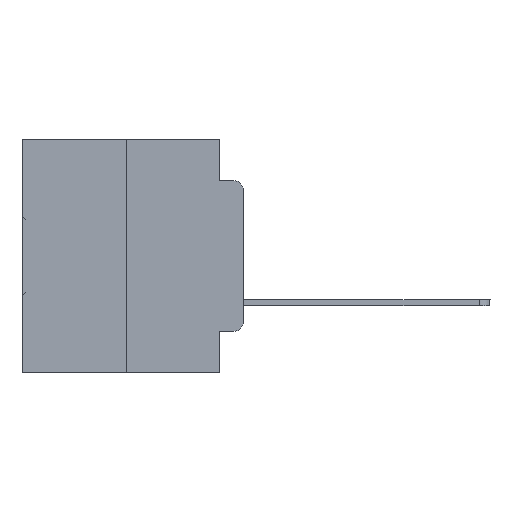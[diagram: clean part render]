
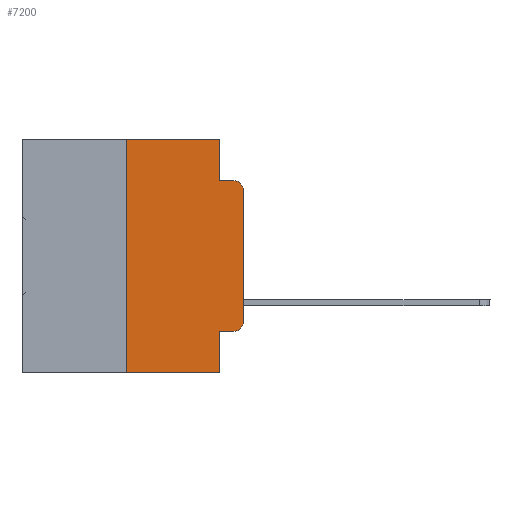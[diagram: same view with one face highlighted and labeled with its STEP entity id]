
A CAD part, left-side view. The second image highlights one B-rep face of the part: STEP entity #7200.
In plain terms, the highlighted planar face has unit normal (-1, 0, 0).
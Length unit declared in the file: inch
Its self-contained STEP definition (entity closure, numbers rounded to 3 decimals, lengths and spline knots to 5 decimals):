
#380 = DIRECTION ( 'NONE',  ( 0., 0., -1. ) ) ;
#623 = VECTOR ( 'NONE', #21628, 39.37008 ) ;
#686 = CARTESIAN_POINT ( 'NONE',  ( 0., 0.02, -0.3915 ) ) ;
#1018 = ORIENTED_EDGE ( 'NONE', *, *, #17901, .F. ) ;
#1447 = DIRECTION ( 'NONE',  ( 0., -1., 0. ) ) ;
#1550 = FACE_OUTER_BOUND ( 'NONE', #14288, .T. ) ;
#1803 = CARTESIAN_POINT ( 'NONE',  ( 0., 0.051, -0.4115 ) ) ;
#2067 = DIRECTION ( 'NONE',  ( 0., 0., -1. ) ) ;
#2581 = CARTESIAN_POINT ( 'NONE',  ( 0., 0.051, 0. ) ) ;
#2599 = CARTESIAN_POINT ( 'NONE',  ( 0., 0.051, 0. ) ) ;
#2606 = CARTESIAN_POINT ( 'NONE',  ( 0., 0.051, -0.0885 ) ) ;
#2809 = VERTEX_POINT ( 'NONE', #28054 ) ;
#3084 = DIRECTION ( 'NONE',  ( -1., 0., 0. ) ) ;
#3842 = CARTESIAN_POINT ( 'NONE',  ( 0., 0., -0.3915 ) ) ;
#4017 = EDGE_CURVE ( 'NONE', #8061, #31795, #25073, .T. ) ;
#4572 = DIRECTION ( 'NONE',  ( 1., 0., 0. ) ) ;
#4584 = EDGE_CURVE ( 'NONE', #8061, #24535, #31628, .T. ) ;
#4909 = CARTESIAN_POINT ( 'NONE',  ( 0., 0.473, 0. ) ) ;
#5187 = LINE ( 'NONE', #12226, #9756 ) ;
#5697 = ORIENTED_EDGE ( 'NONE', *, *, #12408, .T. ) ;
#5806 = CARTESIAN_POINT ( 'NONE',  ( 0., 0.473, -0.5 ) ) ;
#6037 = EDGE_CURVE ( 'NONE', #8994, #27516, #20230, .T. ) ;
#6331 = CARTESIAN_POINT ( 'NONE',  ( 0., 0.051, -0.4115 ) ) ;
#7171 = EDGE_CURVE ( 'NONE', #12189, #2809, #15209, .T. ) ;
#7200 = ADVANCED_FACE ( 'NONE', ( #1550 ), #25599, .F. ) ;
#7308 = CARTESIAN_POINT ( 'NONE',  ( 0., 0.051, 0. ) ) ;
#7859 = ORIENTED_EDGE ( 'NONE', *, *, #6037, .F. ) ;
#8061 = VERTEX_POINT ( 'NONE', #6331 ) ;
#8823 = ORIENTED_EDGE ( 'NONE', *, *, #29715, .F. ) ;
#8994 = VERTEX_POINT ( 'NONE', #2599 ) ;
#9609 = CIRCLE ( 'NONE', #23809, 0.02 ) ;
#9756 = VECTOR ( 'NONE', #14757, 39.37008 ) ;
#9885 = DIRECTION ( 'NONE',  ( 0., 0., 1. ) ) ;
#11040 = VECTOR ( 'NONE', #1447, 39.37008 ) ;
#11096 = CARTESIAN_POINT ( 'NONE',  ( 0., 0.051, -0.5 ) ) ;
#11649 = ORIENTED_EDGE ( 'NONE', *, *, #7171, .T. ) ;
#12012 = ORIENTED_EDGE ( 'NONE', *, *, #4584, .F. ) ;
#12189 = VERTEX_POINT ( 'NONE', #30279 ) ;
#12226 = CARTESIAN_POINT ( 'NONE',  ( 0., 0.25, 0. ) ) ;
#12408 = EDGE_CURVE ( 'NONE', #15533, #12189, #27137, .T. ) ;
#13996 = CARTESIAN_POINT ( 'NONE',  ( 0., 0.25, 0. ) ) ;
#14288 = EDGE_LOOP ( 'NONE', ( #5697, #11649, #30244, #7859, #8823, #1018, #22635, #12012, #19996, #14322 ) ) ;
#14322 = ORIENTED_EDGE ( 'NONE', *, *, #24398, .T. ) ;
#14585 = VERTEX_POINT ( 'NONE', #13996 ) ;
#14757 = DIRECTION ( 'NONE',  ( 0., 0., 1. ) ) ;
#15209 = CIRCLE ( 'NONE', #17328, 0.02 ) ;
#15533 = VERTEX_POINT ( 'NONE', #3842 ) ;
#16756 = EDGE_CURVE ( 'NONE', #33252, #24535, #29791, .T. ) ;
#17328 = AXIS2_PLACEMENT_3D ( 'NONE', #28610, #18133, #28371 ) ;
#17901 = EDGE_CURVE ( 'NONE', #33252, #14585, #5187, .T. ) ;
#18133 = DIRECTION ( 'NONE',  ( -1., 0., 0. ) ) ;
#18257 = EDGE_CURVE ( 'NONE', #27516, #2809, #27036, .T. ) ;
#18319 = CARTESIAN_POINT ( 'NONE',  ( 0., 0.473, 0. ) ) ;
#19069 = AXIS2_PLACEMENT_3D ( 'NONE', #4909, #4572, #2067 ) ;
#19996 = ORIENTED_EDGE ( 'NONE', *, *, #4017, .T. ) ;
#20225 = VECTOR ( 'NONE', #31537, 39.37008 ) ;
#20230 = LINE ( 'NONE', #2581, #26422 ) ;
#21628 = DIRECTION ( 'NONE',  ( 0., -1., 0. ) ) ;
#21705 = VECTOR ( 'NONE', #33289, 39.37008 ) ;
#22635 = ORIENTED_EDGE ( 'NONE', *, *, #16756, .T. ) ;
#23809 = AXIS2_PLACEMENT_3D ( 'NONE', #686, #3084, #32285 ) ;
#24174 = DIRECTION ( 'NONE',  ( 0., -1., 0. ) ) ;
#24398 = EDGE_CURVE ( 'NONE', #31795, #15533, #9609, .T. ) ;
#24535 = VERTEX_POINT ( 'NONE', #11096 ) ;
#25073 = LINE ( 'NONE', #1803, #11040 ) ;
#25108 = VECTOR ( 'NONE', #9885, 39.37008 ) ;
#25126 = CARTESIAN_POINT ( 'NONE',  ( 0., 0.02, -0.4115 ) ) ;
#25599 = PLANE ( 'NONE',  #19069 ) ;
#26422 = VECTOR ( 'NONE', #380, 39.37008 ) ;
#26885 = VECTOR ( 'NONE', #24174, 39.37008 ) ;
#27036 = LINE ( 'NONE', #2606, #623 ) ;
#27137 = LINE ( 'NONE', #28461, #25108 ) ;
#27516 = VERTEX_POINT ( 'NONE', #31226 ) ;
#28054 = CARTESIAN_POINT ( 'NONE',  ( 0., 0.02, -0.0885 ) ) ;
#28371 = DIRECTION ( 'NONE',  ( 0., 0., -1. ) ) ;
#28461 = CARTESIAN_POINT ( 'NONE',  ( 0., 0., 0. ) ) ;
#28610 = CARTESIAN_POINT ( 'NONE',  ( 0., 0.02, -0.1085 ) ) ;
#29715 = EDGE_CURVE ( 'NONE', #14585, #8994, #30122, .T. ) ;
#29791 = LINE ( 'NONE', #5806, #26885 ) ;
#30122 = LINE ( 'NONE', #18319, #20225 ) ;
#30244 = ORIENTED_EDGE ( 'NONE', *, *, #18257, .F. ) ;
#30279 = CARTESIAN_POINT ( 'NONE',  ( 0., 0., -0.1085 ) ) ;
#31226 = CARTESIAN_POINT ( 'NONE',  ( 0., 0.051, -0.0885 ) ) ;
#31537 = DIRECTION ( 'NONE',  ( 0., -1., 0. ) ) ;
#31628 = LINE ( 'NONE', #7308, #21705 ) ;
#31795 = VERTEX_POINT ( 'NONE', #25126 ) ;
#32285 = DIRECTION ( 'NONE',  ( 0., 0., -1. ) ) ;
#32583 = CARTESIAN_POINT ( 'NONE',  ( 0., 0.25, -0.5 ) ) ;
#33252 = VERTEX_POINT ( 'NONE', #32583 ) ;
#33289 = DIRECTION ( 'NONE',  ( 0., 0., -1. ) ) ;
